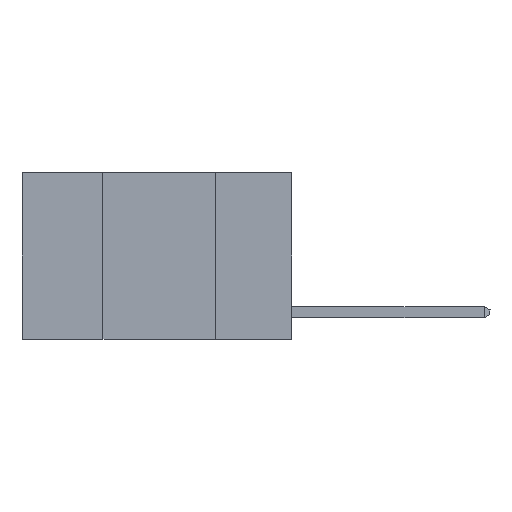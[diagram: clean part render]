
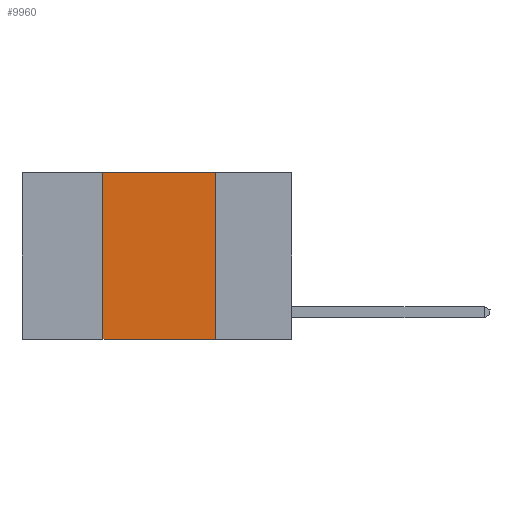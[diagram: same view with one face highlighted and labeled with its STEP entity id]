
A CAD part, left-side view. The second image highlights one B-rep face of the part: STEP entity #9960.
In plain terms, the highlighted planar face has unit normal (-1, 0, 0).
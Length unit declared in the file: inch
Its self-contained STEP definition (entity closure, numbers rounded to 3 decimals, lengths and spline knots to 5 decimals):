
#208 = CARTESIAN_POINT ( 'NONE',  ( 0., 0.17, -0.37 ) ) ;
#270 = DIRECTION ( 'NONE',  ( 0., 0., 1. ) ) ;
#800 = LINE ( 'NONE', #6625, #6118 ) ;
#1869 = DIRECTION ( 'NONE',  ( 0., 0., -1. ) ) ;
#2067 = LINE ( 'NONE', #10420, #12043 ) ;
#2342 = LINE ( 'NONE', #11318, #9616 ) ;
#3111 = ORIENTED_EDGE ( 'NONE', *, *, #6355, .F. ) ;
#3632 = VERTEX_POINT ( 'NONE', #208 ) ;
#3698 = DIRECTION ( 'NONE',  ( 0., -1., 0. ) ) ;
#4155 = CARTESIAN_POINT ( 'NONE',  ( 0., 0.42, 0. ) ) ;
#4274 = AXIS2_PLACEMENT_3D ( 'NONE', #5670, #10692, #1869 ) ;
#4330 = LINE ( 'NONE', #6356, #6294 ) ;
#5608 = DIRECTION ( 'NONE',  ( 0., 0., -1. ) ) ;
#5670 = CARTESIAN_POINT ( 'NONE',  ( 0., 0.6, 0. ) ) ;
#6118 = VECTOR ( 'NONE', #7602, 39.37008 ) ;
#6294 = VECTOR ( 'NONE', #270, 39.37008 ) ;
#6355 = EDGE_CURVE ( 'NONE', #7554, #10917, #800, .T. ) ;
#6356 = CARTESIAN_POINT ( 'NONE',  ( 0., 0.42, 0. ) ) ;
#6416 = FACE_OUTER_BOUND ( 'NONE', #8105, .T. ) ;
#6625 = CARTESIAN_POINT ( 'NONE',  ( 0., 0.6, 0. ) ) ;
#6666 = ORIENTED_EDGE ( 'NONE', *, *, #11619, .T. ) ;
#7554 = VERTEX_POINT ( 'NONE', #4155 ) ;
#7602 = DIRECTION ( 'NONE',  ( 0., -1., 0. ) ) ;
#8105 = EDGE_LOOP ( 'NONE', ( #10984, #3111, #8642, #6666 ) ) ;
#8642 = ORIENTED_EDGE ( 'NONE', *, *, #10573, .F. ) ;
#9616 = VECTOR ( 'NONE', #3698, 39.37008 ) ;
#9960 = ADVANCED_FACE ( 'NONE', ( #6416 ), #10563, .F. ) ;
#10420 = CARTESIAN_POINT ( 'NONE',  ( 0., 0.17, 0. ) ) ;
#10460 = VERTEX_POINT ( 'NONE', #12472 ) ;
#10481 = EDGE_CURVE ( 'NONE', #10917, #3632, #2067, .T. ) ;
#10563 = PLANE ( 'NONE',  #4274 ) ;
#10573 = EDGE_CURVE ( 'NONE', #10460, #7554, #4330, .T. ) ;
#10671 = CARTESIAN_POINT ( 'NONE',  ( 0., 0.17, 0. ) ) ;
#10692 = DIRECTION ( 'NONE',  ( 1., 0., 0. ) ) ;
#10917 = VERTEX_POINT ( 'NONE', #10671 ) ;
#10984 = ORIENTED_EDGE ( 'NONE', *, *, #10481, .F. ) ;
#11318 = CARTESIAN_POINT ( 'NONE',  ( 0., 0.6, -0.37 ) ) ;
#11619 = EDGE_CURVE ( 'NONE', #10460, #3632, #2342, .T. ) ;
#12043 = VECTOR ( 'NONE', #5608, 39.37008 ) ;
#12472 = CARTESIAN_POINT ( 'NONE',  ( 0., 0.42, -0.37 ) ) ;
